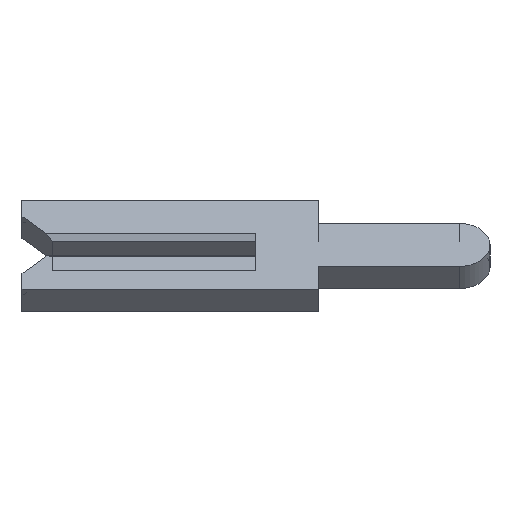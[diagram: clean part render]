
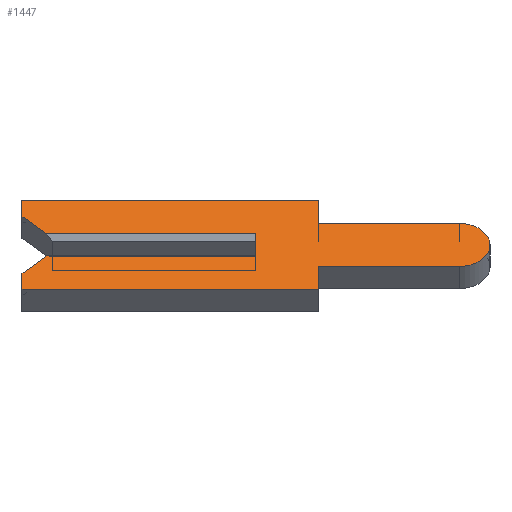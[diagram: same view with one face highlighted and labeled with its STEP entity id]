
A CAD part, left-side view. The second image highlights one B-rep face of the part: STEP entity #1447.
In plain terms, the highlighted face is planar.
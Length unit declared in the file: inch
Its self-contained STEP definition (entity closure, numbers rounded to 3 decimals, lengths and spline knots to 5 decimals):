
#16 = AXIS2_PLACEMENT_3D ( 'NONE', #244, #1750, #2168 ) ;
#22 = ORIENTED_EDGE ( 'NONE', *, *, #2311, .F. ) ;
#41 = VECTOR ( 'NONE', #1542, 39.37008 ) ;
#96 = ORIENTED_EDGE ( 'NONE', *, *, #1832, .T. ) ;
#112 = LINE ( 'NONE', #1651, #1138 ) ;
#154 = ORIENTED_EDGE ( 'NONE', *, *, #1721, .F. ) ;
#157 = CARTESIAN_POINT ( 'NONE',  ( -0.01, 0.1305, -0.0065 ) ) ;
#171 = EDGE_CURVE ( 'NONE', #1050, #387, #274, .T. ) ;
#213 = VECTOR ( 'NONE', #1840, 39.37008 ) ;
#240 = LINE ( 'NONE', #1622, #2654 ) ;
#244 = CARTESIAN_POINT ( 'NONE',  ( -0.01, -0.1305, 0. ) ) ;
#274 = LINE ( 'NONE', #2305, #1701 ) ;
#309 = LINE ( 'NONE', #2261, #2522 ) ;
#312 = DIRECTION ( 'NONE',  ( 0., 0., -1. ) ) ;
#351 = CARTESIAN_POINT ( 'NONE',  ( -0.01, -0.04, 0.0195 ) ) ;
#371 = LINE ( 'NONE', #157, #2444 ) ;
#373 = CARTESIAN_POINT ( 'NONE',  ( -0.01, 0.15, -0.026 ) ) ;
#376 = CARTESIAN_POINT ( 'NONE',  ( -0.01, -0.1305, -0.0195 ) ) ;
#387 = VERTEX_POINT ( 'NONE', #778 ) ;
#415 = VERTEX_POINT ( 'NONE', #2477 ) ;
#417 = ORIENTED_EDGE ( 'NONE', *, *, #937, .F. ) ;
#418 = VERTEX_POINT ( 'NONE', #373 ) ;
#436 = LINE ( 'NONE', #1628, #2114 ) ;
#466 = CARTESIAN_POINT ( 'NONE',  ( -0.01, 0.134, -0.01 ) ) ;
#522 = VERTEX_POINT ( 'NONE', #986 ) ;
#530 = VERTEX_POINT ( 'NONE', #351 ) ;
#555 = CARTESIAN_POINT ( 'NONE',  ( -0.01, 0.1305, 0.0065 ) ) ;
#564 = VERTEX_POINT ( 'NONE', #1217 ) ;
#584 = VECTOR ( 'NONE', #2299, 39.37008 ) ;
#616 = LINE ( 'NONE', #555, #2287 ) ;
#662 = DIRECTION ( 'NONE',  ( 0., -1., 0. ) ) ;
#743 = VECTOR ( 'NONE', #1591, 39.37008 ) ;
#744 = PLANE ( 'NONE',  #2358 ) ;
#766 = EDGE_CURVE ( 'NONE', #387, #530, #436, .T. ) ;
#778 = CARTESIAN_POINT ( 'NONE',  ( -0.01, -0.04, 0.04 ) ) ;
#782 = EDGE_CURVE ( 'NONE', #522, #2383, #309, .T. ) ;
#937 = EDGE_CURVE ( 'NONE', #530, #1342, #2623, .T. ) ;
#947 = VERTEX_POINT ( 'NONE', #2154 ) ;
#986 = CARTESIAN_POINT ( 'NONE',  ( -0.01, -0.04, -0.0195 ) ) ;
#998 = CARTESIAN_POINT ( 'NONE',  ( -0.01, -0.04, 0.0195 ) ) ;
#1000 = LINE ( 'NONE', #1170, #743 ) ;
#1050 = VERTEX_POINT ( 'NONE', #2366 ) ;
#1085 = EDGE_LOOP ( 'NONE', ( #96, #1857, #22, #2423, #2020, #154, #1466, #1327, #2323, #417, #2010, #1427, #2530, #2129 ) ) ;
#1138 = VECTOR ( 'NONE', #1660, 39.37008 ) ;
#1155 = CARTESIAN_POINT ( 'NONE',  ( -0.01, -0.1305, 0. ) ) ;
#1170 = CARTESIAN_POINT ( 'NONE',  ( -0.01, -0.04, -0.0195 ) ) ;
#1217 = CARTESIAN_POINT ( 'NONE',  ( -0.01, 0.134, 0.01 ) ) ;
#1245 = EDGE_CURVE ( 'NONE', #947, #418, #1311, .T. ) ;
#1248 = CARTESIAN_POINT ( 'NONE',  ( -0.01, 0., -0.01 ) ) ;
#1311 = LINE ( 'NONE', #1661, #584 ) ;
#1327 = ORIENTED_EDGE ( 'NONE', *, *, #1411, .F. ) ;
#1342 = VERTEX_POINT ( 'NONE', #2573 ) ;
#1376 = VECTOR ( 'NONE', #662, 39.37008 ) ;
#1411 = EDGE_CURVE ( 'NONE', #2571, #522, #1000, .T. ) ;
#1427 = ORIENTED_EDGE ( 'NONE', *, *, #171, .F. ) ;
#1431 = DIRECTION ( 'NONE',  ( 0., 0., 1. ) ) ;
#1447 = ADVANCED_FACE ( 'NONE', ( #2082 ), #744, .F. ) ;
#1463 = VERTEX_POINT ( 'NONE', #466 ) ;
#1466 = ORIENTED_EDGE ( 'NONE', *, *, #782, .F. ) ;
#1521 = CARTESIAN_POINT ( 'NONE',  ( -0.01, 0.15, -0.04 ) ) ;
#1542 = DIRECTION ( 'NONE',  ( 0., -1., 0. ) ) ;
#1570 = LINE ( 'NONE', #1806, #41 ) ;
#1591 = DIRECTION ( 'NONE',  ( 0., 1., 0. ) ) ;
#1606 = LINE ( 'NONE', #1521, #1670 ) ;
#1613 = CARTESIAN_POINT ( 'NONE',  ( -0.01, -0.1305, -0.01 ) ) ;
#1622 = CARTESIAN_POINT ( 'NONE',  ( -0.01, 0.15, 0.026 ) ) ;
#1628 = CARTESIAN_POINT ( 'NONE',  ( -0.01, -0.04, 0.04 ) ) ;
#1651 = CARTESIAN_POINT ( 'NONE',  ( -0.01, 0., 0.0065 ) ) ;
#1660 = DIRECTION ( 'NONE',  ( 0., 0., 1. ) ) ;
#1661 = CARTESIAN_POINT ( 'NONE',  ( -0.01, 0.15, -0.026 ) ) ;
#1670 = VECTOR ( 'NONE', #1968, 39.37008 ) ;
#1701 = VECTOR ( 'NONE', #2554, 39.37008 ) ;
#1721 = EDGE_CURVE ( 'NONE', #2383, #947, #1606, .T. ) ;
#1750 = DIRECTION ( 'NONE',  ( 1., 0., 0. ) ) ;
#1796 = EDGE_CURVE ( 'NONE', #1342, #2571, #2144, .T. ) ;
#1806 = CARTESIAN_POINT ( 'NONE',  ( -0.01, 0.15, 0.01 ) ) ;
#1832 = EDGE_CURVE ( 'NONE', #564, #2350, #1570, .T. ) ;
#1840 = DIRECTION ( 'NONE',  ( 0., -1., 0. ) ) ;
#1857 = ORIENTED_EDGE ( 'NONE', *, *, #2547, .F. ) ;
#1923 = DIRECTION ( 'NONE',  ( 0., 0., -1. ) ) ;
#1968 = DIRECTION ( 'NONE',  ( 0., 1., 0. ) ) ;
#1974 = EDGE_CURVE ( 'NONE', #415, #1050, #240, .T. ) ;
#2010 = ORIENTED_EDGE ( 'NONE', *, *, #766, .F. ) ;
#2020 = ORIENTED_EDGE ( 'NONE', *, *, #1245, .F. ) ;
#2044 = DIRECTION ( 'NONE',  ( 0., 0.707, 0.707 ) ) ;
#2072 = EDGE_CURVE ( 'NONE', #418, #1463, #371, .T. ) ;
#2073 = DIRECTION ( 'NONE',  ( 0., 0., -1. ) ) ;
#2082 = FACE_OUTER_BOUND ( 'NONE', #1085, .T. ) ;
#2114 = VECTOR ( 'NONE', #2073, 39.37008 ) ;
#2129 = ORIENTED_EDGE ( 'NONE', *, *, #2272, .F. ) ;
#2144 = CIRCLE ( 'NONE', #16, 0.0195 ) ;
#2154 = CARTESIAN_POINT ( 'NONE',  ( -0.01, 0.15, -0.04 ) ) ;
#2168 = DIRECTION ( 'NONE',  ( 0., 0., -1. ) ) ;
#2258 = CARTESIAN_POINT ( 'NONE',  ( -0.01, -0.04, -0.04 ) ) ;
#2261 = CARTESIAN_POINT ( 'NONE',  ( -0.01, -0.04, -0.04 ) ) ;
#2272 = EDGE_CURVE ( 'NONE', #564, #415, #616, .T. ) ;
#2287 = VECTOR ( 'NONE', #2044, 39.37008 ) ;
#2299 = DIRECTION ( 'NONE',  ( 0., 0., 1. ) ) ;
#2305 = CARTESIAN_POINT ( 'NONE',  ( -0.01, 0.15, 0.04 ) ) ;
#2311 = EDGE_CURVE ( 'NONE', #1463, #2537, #2413, .T. ) ;
#2323 = ORIENTED_EDGE ( 'NONE', *, *, #1796, .F. ) ;
#2350 = VERTEX_POINT ( 'NONE', #2483 ) ;
#2358 = AXIS2_PLACEMENT_3D ( 'NONE', #1155, #2389, #312 ) ;
#2366 = CARTESIAN_POINT ( 'NONE',  ( -0.01, 0.15, 0.04 ) ) ;
#2383 = VERTEX_POINT ( 'NONE', #2258 ) ;
#2389 = DIRECTION ( 'NONE',  ( 1., 0., 0. ) ) ;
#2413 = LINE ( 'NONE', #1613, #213 ) ;
#2423 = ORIENTED_EDGE ( 'NONE', *, *, #2072, .F. ) ;
#2444 = VECTOR ( 'NONE', #2492, 39.37008 ) ;
#2477 = CARTESIAN_POINT ( 'NONE',  ( -0.01, 0.15, 0.026 ) ) ;
#2483 = CARTESIAN_POINT ( 'NONE',  ( -0.01, 0., 0.01 ) ) ;
#2492 = DIRECTION ( 'NONE',  ( 0., -0.707, 0.707 ) ) ;
#2522 = VECTOR ( 'NONE', #1923, 39.37008 ) ;
#2530 = ORIENTED_EDGE ( 'NONE', *, *, #1974, .F. ) ;
#2537 = VERTEX_POINT ( 'NONE', #1248 ) ;
#2547 = EDGE_CURVE ( 'NONE', #2537, #2350, #112, .T. ) ;
#2554 = DIRECTION ( 'NONE',  ( 0., -1., 0. ) ) ;
#2571 = VERTEX_POINT ( 'NONE', #376 ) ;
#2573 = CARTESIAN_POINT ( 'NONE',  ( -0.01, -0.1305, 0.0195 ) ) ;
#2623 = LINE ( 'NONE', #998, #1376 ) ;
#2654 = VECTOR ( 'NONE', #1431, 39.37008 ) ;
